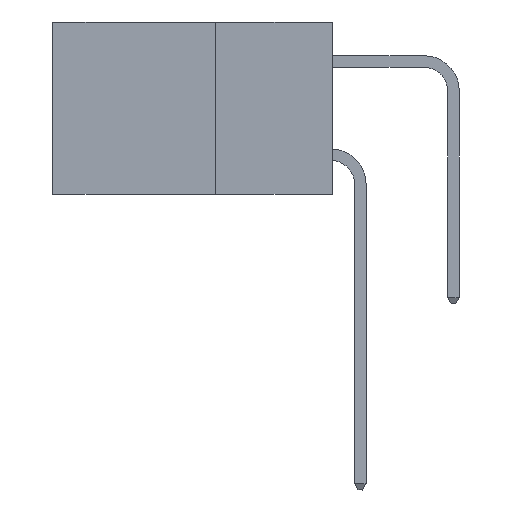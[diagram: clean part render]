
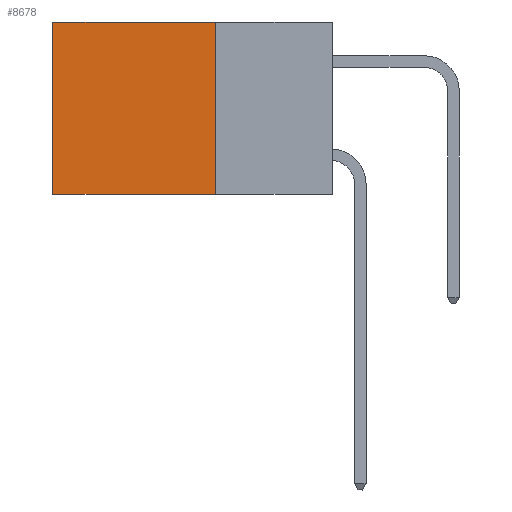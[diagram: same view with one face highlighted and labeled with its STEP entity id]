
A CAD part, left-side view. The second image highlights one B-rep face of the part: STEP entity #8678.
In plain terms, the highlighted planar face has unit normal (-1, 0, 0).
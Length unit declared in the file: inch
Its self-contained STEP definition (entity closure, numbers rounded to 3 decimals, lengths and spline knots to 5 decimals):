
#81 = ORIENTED_EDGE ( 'NONE', *, *, #14806, .F. ) ;
#185 = EDGE_CURVE ( 'NONE', #3609, #3086, #6917, .T. ) ;
#1339 = CARTESIAN_POINT ( 'NONE',  ( 0.298, 0.25, 0. ) ) ;
#1557 = EDGE_CURVE ( 'NONE', #12726, #4515, #14789, .T. ) ;
#1667 = CARTESIAN_POINT ( 'NONE',  ( 0.298, 0.25, -0.37 ) ) ;
#1832 = CARTESIAN_POINT ( 'NONE',  ( 0.298, 0.6, -0.37 ) ) ;
#2034 = DIRECTION ( 'NONE',  ( 0., 0., -1. ) ) ;
#2568 = VECTOR ( 'NONE', #2784, 39.37008 ) ;
#2784 = DIRECTION ( 'NONE',  ( 0., 1., 0. ) ) ;
#2935 = CARTESIAN_POINT ( 'NONE',  ( 0.298, 0.25, 0. ) ) ;
#3086 = VERTEX_POINT ( 'NONE', #1832 ) ;
#3138 = DIRECTION ( 'NONE',  ( 0., 1., 0. ) ) ;
#3609 = VERTEX_POINT ( 'NONE', #1667 ) ;
#4515 = VERTEX_POINT ( 'NONE', #5406 ) ;
#4786 = AXIS2_PLACEMENT_3D ( 'NONE', #15259, #5611, #2034 ) ;
#5303 = ORIENTED_EDGE ( 'NONE', *, *, #1557, .T. ) ;
#5406 = CARTESIAN_POINT ( 'NONE',  ( 0.298, 0.6, 0. ) ) ;
#5611 = DIRECTION ( 'NONE',  ( 1., 0., 0. ) ) ;
#6917 = LINE ( 'NONE', #10465, #14994 ) ;
#7858 = CARTESIAN_POINT ( 'NONE',  ( 0.298, 0.6, 0. ) ) ;
#7963 = PLANE ( 'NONE',  #4786 ) ;
#8494 = VECTOR ( 'NONE', #10932, 39.37008 ) ;
#8678 = ADVANCED_FACE ( 'NONE', ( #8866 ), #7963, .F. ) ;
#8866 = FACE_OUTER_BOUND ( 'NONE', #9599, .T. ) ;
#8879 = ORIENTED_EDGE ( 'NONE', *, *, #11951, .T. ) ;
#9599 = EDGE_LOOP ( 'NONE', ( #8879, #15460, #81, #5303 ) ) ;
#9663 = VECTOR ( 'NONE', #15207, 39.37008 ) ;
#10465 = CARTESIAN_POINT ( 'NONE',  ( 0.298, 0.25, -0.37 ) ) ;
#10932 = DIRECTION ( 'NONE',  ( 0., 0., -1. ) ) ;
#11762 = LINE ( 'NONE', #7858, #9663 ) ;
#11951 = EDGE_CURVE ( 'NONE', #4515, #3086, #11762, .T. ) ;
#12726 = VERTEX_POINT ( 'NONE', #1339 ) ;
#14445 = CARTESIAN_POINT ( 'NONE',  ( 0.298, 0.25, 0. ) ) ;
#14789 = LINE ( 'NONE', #2935, #2568 ) ;
#14806 = EDGE_CURVE ( 'NONE', #12726, #3609, #15265, .T. ) ;
#14994 = VECTOR ( 'NONE', #3138, 39.37008 ) ;
#15207 = DIRECTION ( 'NONE',  ( 0., 0., -1. ) ) ;
#15259 = CARTESIAN_POINT ( 'NONE',  ( 0.298, 0.25, 0. ) ) ;
#15265 = LINE ( 'NONE', #14445, #8494 ) ;
#15460 = ORIENTED_EDGE ( 'NONE', *, *, #185, .F. ) ;
